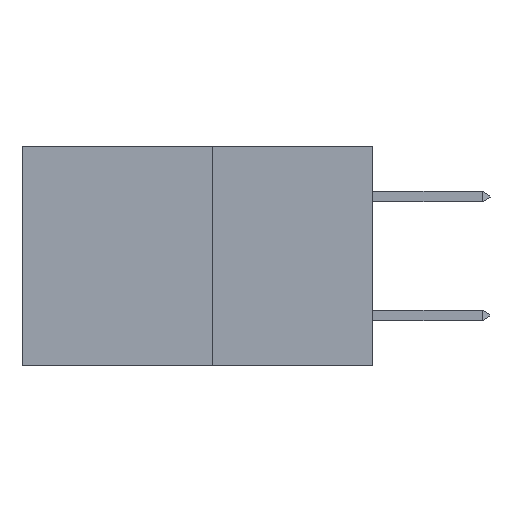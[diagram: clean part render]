
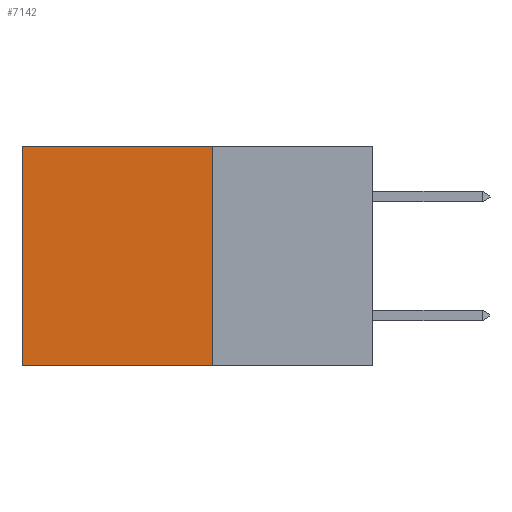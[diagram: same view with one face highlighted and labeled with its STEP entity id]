
A CAD part, left-side view. The second image highlights one B-rep face of the part: STEP entity #7142.
In plain terms, the highlighted planar face has unit normal (-1, 0, 0).
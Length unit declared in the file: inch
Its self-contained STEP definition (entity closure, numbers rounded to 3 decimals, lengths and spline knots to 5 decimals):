
#572 = CARTESIAN_POINT ( 'NONE',  ( 0.277, 0.27, 0. ) ) ;
#601 = ORIENTED_EDGE ( 'NONE', *, *, #1619, .F. ) ;
#678 = LINE ( 'NONE', #9905, #11509 ) ;
#726 = DIRECTION ( 'NONE',  ( 1., 0., 0. ) ) ;
#1605 = VERTEX_POINT ( 'NONE', #1724 ) ;
#1619 = EDGE_CURVE ( 'NONE', #12529, #8940, #12003, .T. ) ;
#1724 = CARTESIAN_POINT ( 'NONE',  ( 0.277, 0.59, 0. ) ) ;
#1984 = VECTOR ( 'NONE', #8794, 39.37008 ) ;
#2655 = CARTESIAN_POINT ( 'NONE',  ( 0.277, 0.27, -0.37 ) ) ;
#3455 = ORIENTED_EDGE ( 'NONE', *, *, #7150, .F. ) ;
#3928 = DIRECTION ( 'NONE',  ( 0., 0., -1. ) ) ;
#4029 = EDGE_LOOP ( 'NONE', ( #13139, #601, #3455, #9086 ) ) ;
#4504 = LINE ( 'NONE', #6802, #9159 ) ;
#4697 = CARTESIAN_POINT ( 'NONE',  ( 0.277, 0.59, -0.37 ) ) ;
#4909 = PLANE ( 'NONE',  #11435 ) ;
#4969 = VECTOR ( 'NONE', #6113, 39.37008 ) ;
#5060 = LINE ( 'NONE', #572, #1984 ) ;
#5106 = CARTESIAN_POINT ( 'NONE',  ( 0.277, 0.27, -0.37 ) ) ;
#5879 = CARTESIAN_POINT ( 'NONE',  ( 0.277, 0.27, -0.37 ) ) ;
#6113 = DIRECTION ( 'NONE',  ( 0., 1., 0. ) ) ;
#6170 = FACE_OUTER_BOUND ( 'NONE', #4029, .T. ) ;
#6802 = CARTESIAN_POINT ( 'NONE',  ( 0.277, 0.59, -0.37 ) ) ;
#7142 = ADVANCED_FACE ( 'NONE', ( #6170 ), #4909, .F. ) ;
#7150 = EDGE_CURVE ( 'NONE', #12002, #12529, #678, .T. ) ;
#7797 = EDGE_CURVE ( 'NONE', #12002, #1605, #5060, .T. ) ;
#7807 = DIRECTION ( 'NONE',  ( 0., 0., -1. ) ) ;
#7916 = DIRECTION ( 'NONE',  ( 0., 0., -1. ) ) ;
#8794 = DIRECTION ( 'NONE',  ( 0., 1., 0. ) ) ;
#8940 = VERTEX_POINT ( 'NONE', #4697 ) ;
#9086 = ORIENTED_EDGE ( 'NONE', *, *, #7797, .T. ) ;
#9159 = VECTOR ( 'NONE', #7807, 39.37008 ) ;
#9905 = CARTESIAN_POINT ( 'NONE',  ( 0.277, 0.27, -0.37 ) ) ;
#11435 = AXIS2_PLACEMENT_3D ( 'NONE', #5879, #726, #7916 ) ;
#11509 = VECTOR ( 'NONE', #3928, 39.37008 ) ;
#12002 = VERTEX_POINT ( 'NONE', #13045 ) ;
#12003 = LINE ( 'NONE', #5106, #4969 ) ;
#12529 = VERTEX_POINT ( 'NONE', #2655 ) ;
#12594 = EDGE_CURVE ( 'NONE', #1605, #8940, #4504, .T. ) ;
#13045 = CARTESIAN_POINT ( 'NONE',  ( 0.277, 0.27, 0. ) ) ;
#13139 = ORIENTED_EDGE ( 'NONE', *, *, #12594, .T. ) ;
